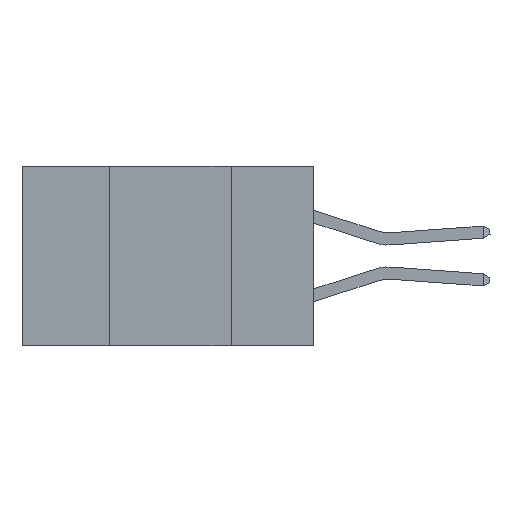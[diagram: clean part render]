
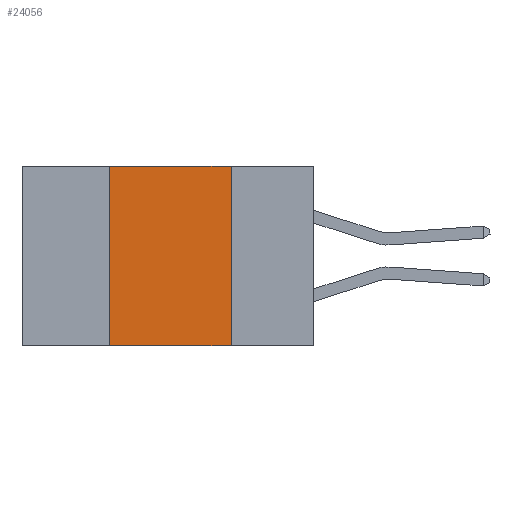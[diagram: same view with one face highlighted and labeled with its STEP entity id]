
A CAD part, left-side view. The second image highlights one B-rep face of the part: STEP entity #24056.
In plain terms, the highlighted planar face has unit normal (-1, 0, 0).
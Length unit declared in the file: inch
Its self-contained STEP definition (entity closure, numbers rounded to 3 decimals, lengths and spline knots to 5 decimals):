
#123 = CARTESIAN_POINT ( 'NONE',  ( 0., 0.42, 0. ) ) ;
#1915 = VERTEX_POINT ( 'NONE', #123 ) ;
#5311 = ORIENTED_EDGE ( 'NONE', *, *, #11189, .F. ) ;
#5864 = DIRECTION ( 'NONE',  ( 0., -1., 0. ) ) ;
#6673 = VECTOR ( 'NONE', #12781, 39.37008 ) ;
#7908 = DIRECTION ( 'NONE',  ( 0., 0., -1. ) ) ;
#9187 = EDGE_CURVE ( 'NONE', #25392, #20019, #30554, .T. ) ;
#9472 = VECTOR ( 'NONE', #5864, 39.37008 ) ;
#9513 = VECTOR ( 'NONE', #33042, 39.37008 ) ;
#10076 = LINE ( 'NONE', #23088, #6673 ) ;
#10719 = CARTESIAN_POINT ( 'NONE',  ( 0., 0.17, -0.37 ) ) ;
#11189 = EDGE_CURVE ( 'NONE', #12561, #20019, #26720, .T. ) ;
#12561 = VERTEX_POINT ( 'NONE', #20986 ) ;
#12781 = DIRECTION ( 'NONE',  ( 0., -1., 0. ) ) ;
#13026 = CARTESIAN_POINT ( 'NONE',  ( 0., 0.17, 0. ) ) ;
#13303 = PLANE ( 'NONE',  #22851 ) ;
#13805 = LINE ( 'NONE', #22115, #9513 ) ;
#13998 = CARTESIAN_POINT ( 'NONE',  ( 0., 0.6, -0.37 ) ) ;
#20019 = VERTEX_POINT ( 'NONE', #10719 ) ;
#20986 = CARTESIAN_POINT ( 'NONE',  ( 0., 0.17, 0. ) ) ;
#21654 = EDGE_LOOP ( 'NONE', ( #5311, #24390, #24708, #25141 ) ) ;
#22115 = CARTESIAN_POINT ( 'NONE',  ( 0., 0.42, 0. ) ) ;
#22398 = VECTOR ( 'NONE', #34798, 39.37008 ) ;
#22851 = AXIS2_PLACEMENT_3D ( 'NONE', #29883, #32547, #7908 ) ;
#23088 = CARTESIAN_POINT ( 'NONE',  ( 0., 0.6, 0. ) ) ;
#24056 = ADVANCED_FACE ( 'NONE', ( #27535 ), #13303, .F. ) ;
#24390 = ORIENTED_EDGE ( 'NONE', *, *, #30285, .F. ) ;
#24708 = ORIENTED_EDGE ( 'NONE', *, *, #31135, .F. ) ;
#25141 = ORIENTED_EDGE ( 'NONE', *, *, #9187, .T. ) ;
#25392 = VERTEX_POINT ( 'NONE', #28870 ) ;
#26720 = LINE ( 'NONE', #13026, #22398 ) ;
#27535 = FACE_OUTER_BOUND ( 'NONE', #21654, .T. ) ;
#28870 = CARTESIAN_POINT ( 'NONE',  ( 0., 0.42, -0.37 ) ) ;
#29883 = CARTESIAN_POINT ( 'NONE',  ( 0., 0.6, 0. ) ) ;
#30285 = EDGE_CURVE ( 'NONE', #1915, #12561, #10076, .T. ) ;
#30554 = LINE ( 'NONE', #13998, #9472 ) ;
#31135 = EDGE_CURVE ( 'NONE', #25392, #1915, #13805, .T. ) ;
#32547 = DIRECTION ( 'NONE',  ( 1., 0., 0. ) ) ;
#33042 = DIRECTION ( 'NONE',  ( 0., 0., 1. ) ) ;
#34798 = DIRECTION ( 'NONE',  ( 0., 0., -1. ) ) ;
